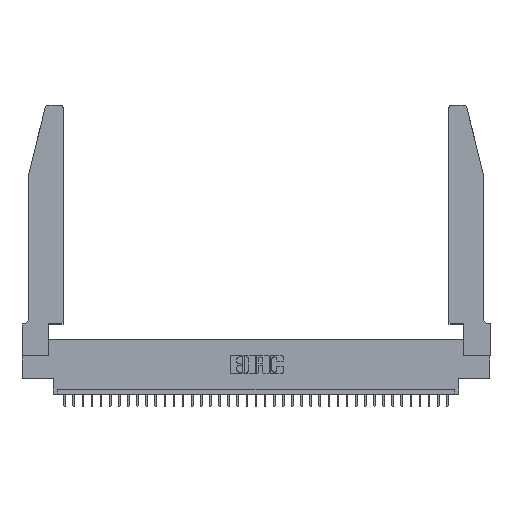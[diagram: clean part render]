
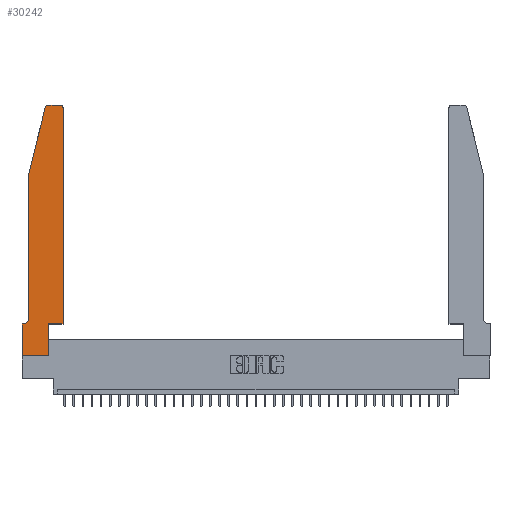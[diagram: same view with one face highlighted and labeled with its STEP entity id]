
A CAD part, top view. The second image highlights one B-rep face of the part: STEP entity #30242.
In plain terms, the highlighted planar face has unit normal (0, 0, 1).
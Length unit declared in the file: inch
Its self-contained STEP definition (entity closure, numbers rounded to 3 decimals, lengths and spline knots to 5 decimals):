
#110 = VECTOR ( 'NONE', #7066, 39.37008 ) ;
#367 = DIRECTION ( 'NONE',  ( 0., 1., 0. ) ) ;
#1168 = VECTOR ( 'NONE', #18555, 39.37008 ) ;
#1472 = VERTEX_POINT ( 'NONE', #14397 ) ;
#2169 = CARTESIAN_POINT ( 'NONE',  ( 0.0755, 0.42, 0.37 ) ) ;
#2373 = LINE ( 'NONE', #13870, #36070 ) ;
#2454 = DIRECTION ( 'NONE',  ( 1., 0., 0. ) ) ;
#3065 = ORIENTED_EDGE ( 'NONE', *, *, #7644, .T. ) ;
#3105 = VERTEX_POINT ( 'NONE', #30638 ) ;
#3680 = CARTESIAN_POINT ( 'NONE',  ( 0.4505, 0.35, 0.37 ) ) ;
#3736 = EDGE_CURVE ( 'NONE', #7338, #9568, #6679, .T. ) ;
#4169 = VERTEX_POINT ( 'NONE', #12861 ) ;
#5131 = CARTESIAN_POINT ( 'NONE',  ( 0.0755, 2., 0.37 ) ) ;
#5522 = AXIS2_PLACEMENT_3D ( 'NONE', #14196, #22846, #8744 ) ;
#5974 = DIRECTION ( 'NONE',  ( 0., 0., 1. ) ) ;
#6679 = LINE ( 'NONE', #3680, #1168 ) ;
#7066 = DIRECTION ( 'NONE',  ( 0., 1., 0. ) ) ;
#7338 = VERTEX_POINT ( 'NONE', #15570 ) ;
#7644 = EDGE_CURVE ( 'NONE', #29081, #8959, #26264, .T. ) ;
#8744 = DIRECTION ( 'NONE',  ( 1., 0., 0. ) ) ;
#8959 = VERTEX_POINT ( 'NONE', #2169 ) ;
#9026 = VECTOR ( 'NONE', #22351, 39.37008 ) ;
#9568 = VERTEX_POINT ( 'NONE', #29412 ) ;
#10011 = ORIENTED_EDGE ( 'NONE', *, *, #16112, .T. ) ;
#10764 = FACE_OUTER_BOUND ( 'NONE', #34914, .T. ) ;
#10776 = EDGE_CURVE ( 'NONE', #12162, #29081, #13440, .T. ) ;
#12162 = VERTEX_POINT ( 'NONE', #28901 ) ;
#12509 = VERTEX_POINT ( 'NONE', #24923 ) ;
#12697 = VECTOR ( 'NONE', #26442, 39.37008 ) ;
#12773 = CIRCLE ( 'NONE', #5522, 0.03 ) ;
#12861 = CARTESIAN_POINT ( 'NONE',  ( 0., 0., 0.37 ) ) ;
#12934 = EDGE_CURVE ( 'NONE', #3105, #7338, #17676, .T. ) ;
#13252 = DIRECTION ( 'NONE',  ( -0.239, -0.971, 0. ) ) ;
#13440 = LINE ( 'NONE', #5131, #14138 ) ;
#13574 = ORIENTED_EDGE ( 'NONE', *, *, #10776, .T. ) ;
#13870 = CARTESIAN_POINT ( 'NONE',  ( 0., 0., 0.37 ) ) ;
#14138 = VECTOR ( 'NONE', #13252, 39.37008 ) ;
#14196 = CARTESIAN_POINT ( 'NONE',  ( 0.284, 2.72, 0.37 ) ) ;
#14397 = CARTESIAN_POINT ( 'NONE',  ( 0.4205, 2.75, 0.37 ) ) ;
#15570 = CARTESIAN_POINT ( 'NONE',  ( 0.2865, 0.35, 0.37 ) ) ;
#15621 = EDGE_CURVE ( 'NONE', #22166, #1472, #18806, .T. ) ;
#16112 = EDGE_CURVE ( 'NONE', #4169, #3105, #30148, .T. ) ;
#16212 = ORIENTED_EDGE ( 'NONE', *, *, #15621, .T. ) ;
#16622 = ORIENTED_EDGE ( 'NONE', *, *, #3736, .T. ) ;
#16742 = CARTESIAN_POINT ( 'NONE',  ( 0.0755, 2., 0.37 ) ) ;
#16774 = ORIENTED_EDGE ( 'NONE', *, *, #31515, .T. ) ;
#16993 = ORIENTED_EDGE ( 'NONE', *, *, #29611, .T. ) ;
#17676 = LINE ( 'NONE', #19759, #34063 ) ;
#18555 = DIRECTION ( 'NONE',  ( 1., 0., 0. ) ) ;
#18806 = CIRCLE ( 'NONE', #23620, 0.03 ) ;
#18867 = CARTESIAN_POINT ( 'NONE',  ( 0., 0., 0.37 ) ) ;
#19759 = CARTESIAN_POINT ( 'NONE',  ( 0.2865, 0.35, 0.37 ) ) ;
#20178 = CARTESIAN_POINT ( 'NONE',  ( 0., 0.35, 0.37 ) ) ;
#20558 = VECTOR ( 'NONE', #30782, 39.37008 ) ;
#21253 = EDGE_CURVE ( 'NONE', #8959, #12509, #29223, .T. ) ;
#21382 = LINE ( 'NONE', #35471, #110 ) ;
#22166 = VERTEX_POINT ( 'NONE', #23845 ) ;
#22305 = AXIS2_PLACEMENT_3D ( 'NONE', #36710, #25622, #2454 ) ;
#22351 = DIRECTION ( 'NONE',  ( -1., 0., 0. ) ) ;
#22523 = CARTESIAN_POINT ( 'NONE',  ( 0.284, 2.75, 0.37 ) ) ;
#22846 = DIRECTION ( 'NONE',  ( 0., 0., 1. ) ) ;
#23019 = CARTESIAN_POINT ( 'NONE',  ( 0.0055, 0.42, 0.37 ) ) ;
#23194 = VERTEX_POINT ( 'NONE', #22523 ) ;
#23203 = DIRECTION ( 'NONE',  ( 0., 0., -1. ) ) ;
#23620 = AXIS2_PLACEMENT_3D ( 'NONE', #25937, #5974, #34423 ) ;
#23845 = CARTESIAN_POINT ( 'NONE',  ( 0.4505, 2.72, 0.37 ) ) ;
#24923 = CARTESIAN_POINT ( 'NONE',  ( 0.0055, 0.35, 0.37 ) ) ;
#25322 = CARTESIAN_POINT ( 'NONE',  ( 0.2605, 2.75, 0.37 ) ) ;
#25341 = DIRECTION ( 'NONE',  ( 0., -1., 0. ) ) ;
#25622 = DIRECTION ( 'NONE',  ( 0., 0., 1. ) ) ;
#25937 = CARTESIAN_POINT ( 'NONE',  ( 0.4205, 2.72, 0.37 ) ) ;
#26264 = LINE ( 'NONE', #35110, #12697 ) ;
#26442 = DIRECTION ( 'NONE',  ( 0., -1., 0. ) ) ;
#26484 = VERTEX_POINT ( 'NONE', #20178 ) ;
#28352 = CARTESIAN_POINT ( 'NONE',  ( 0.0755, 0.35, 0.37 ) ) ;
#28901 = CARTESIAN_POINT ( 'NONE',  ( 0.25487, 2.72718, 0.37 ) ) ;
#29011 = VECTOR ( 'NONE', #30329, 39.37008 ) ;
#29081 = VERTEX_POINT ( 'NONE', #16742 ) ;
#29223 = CIRCLE ( 'NONE', #30994, 0.07 ) ;
#29412 = CARTESIAN_POINT ( 'NONE',  ( 0.4505, 0.35, 0.37 ) ) ;
#29525 = EDGE_CURVE ( 'NONE', #12509, #26484, #33466, .T. ) ;
#29611 = EDGE_CURVE ( 'NONE', #26484, #4169, #2373, .T. ) ;
#30148 = LINE ( 'NONE', #18867, #29011 ) ;
#30242 = ADVANCED_FACE ( 'NONE', ( #10764 ), #31249, .T. ) ;
#30329 = DIRECTION ( 'NONE',  ( 1., 0., 0. ) ) ;
#30354 = ORIENTED_EDGE ( 'NONE', *, *, #31208, .T. ) ;
#30417 = LINE ( 'NONE', #25322, #20558 ) ;
#30638 = CARTESIAN_POINT ( 'NONE',  ( 0.2865, 0., 0.37 ) ) ;
#30782 = DIRECTION ( 'NONE',  ( -1., 0., 0. ) ) ;
#30994 = AXIS2_PLACEMENT_3D ( 'NONE', #23019, #23203, #34686 ) ;
#31208 = EDGE_CURVE ( 'NONE', #1472, #23194, #30417, .T. ) ;
#31249 = PLANE ( 'NONE',  #22305 ) ;
#31515 = EDGE_CURVE ( 'NONE', #9568, #22166, #21382, .T. ) ;
#31770 = EDGE_CURVE ( 'NONE', #23194, #12162, #12773, .T. ) ;
#33466 = LINE ( 'NONE', #28352, #9026 ) ;
#34063 = VECTOR ( 'NONE', #367, 39.37008 ) ;
#34423 = DIRECTION ( 'NONE',  ( 1., 0., 0. ) ) ;
#34686 = DIRECTION ( 'NONE',  ( -1., 0., 0. ) ) ;
#34914 = EDGE_LOOP ( 'NONE', ( #30354, #35565, #13574, #3065, #36417, #35071, #16993, #10011, #37177, #16622, #16774, #16212 ) ) ;
#35071 = ORIENTED_EDGE ( 'NONE', *, *, #29525, .T. ) ;
#35110 = CARTESIAN_POINT ( 'NONE',  ( 0.0755, 2., 0.37 ) ) ;
#35471 = CARTESIAN_POINT ( 'NONE',  ( 0.4505, 0.35, 0.37 ) ) ;
#35565 = ORIENTED_EDGE ( 'NONE', *, *, #31770, .T. ) ;
#36070 = VECTOR ( 'NONE', #25341, 39.37008 ) ;
#36417 = ORIENTED_EDGE ( 'NONE', *, *, #21253, .T. ) ;
#36710 = CARTESIAN_POINT ( 'NONE',  ( 0., 0.35, 0.37 ) ) ;
#37177 = ORIENTED_EDGE ( 'NONE', *, *, #12934, .T. ) ;
